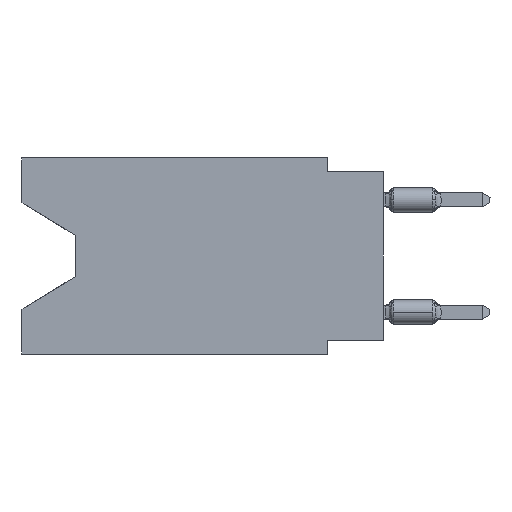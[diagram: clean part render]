
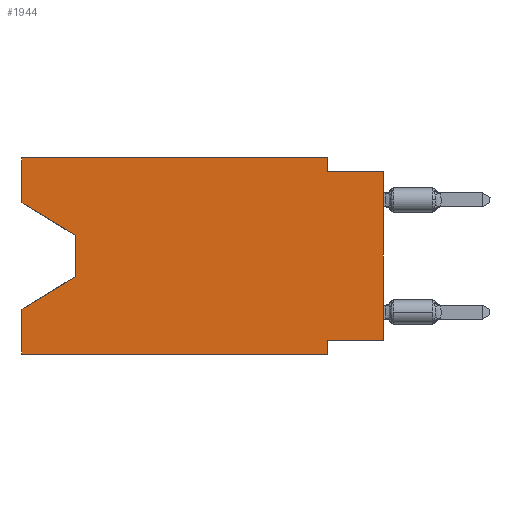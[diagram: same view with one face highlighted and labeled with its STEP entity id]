
A CAD part, left-side view. The second image highlights one B-rep face of the part: STEP entity #1944.
In plain terms, the highlighted planar face has unit normal (-1, 0, 0).
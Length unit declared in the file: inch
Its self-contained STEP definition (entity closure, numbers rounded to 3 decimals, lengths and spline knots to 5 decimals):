
#988 = VERTEX_POINT ( 'NONE', #22899 ) ;
#1447 = ORIENTED_EDGE ( 'NONE', *, *, #24468, .T. ) ;
#1481 = VECTOR ( 'NONE', #27851, 39.37008 ) ;
#1639 = CARTESIAN_POINT ( 'NONE',  ( 0., 0.645, 0. ) ) ;
#1944 = ADVANCED_FACE ( 'NONE', ( #41535 ), #12387, .F. ) ;
#2108 = DIRECTION ( 'NONE',  ( 0., 0., -1. ) ) ;
#2214 = CARTESIAN_POINT ( 'NONE',  ( 0., 0.1, -0.35 ) ) ;
#2319 = DIRECTION ( 'NONE',  ( 0., 0., 1. ) ) ;
#2640 = LINE ( 'NONE', #37544, #3293 ) ;
#3031 = CARTESIAN_POINT ( 'NONE',  ( 0., 0.645, -0.35 ) ) ;
#3290 = CARTESIAN_POINT ( 'NONE',  ( 0., 0.55, -0.212 ) ) ;
#3293 = VECTOR ( 'NONE', #4964, 39.37008 ) ;
#4300 = CARTESIAN_POINT ( 'NONE',  ( 0., 0.645, 0. ) ) ;
#4320 = ORIENTED_EDGE ( 'NONE', *, *, #34400, .T. ) ;
#4796 = VERTEX_POINT ( 'NONE', #3031 ) ;
#4964 = DIRECTION ( 'NONE',  ( 0., 0.855, -0.519 ) ) ;
#5058 = VECTOR ( 'NONE', #33320, 39.37008 ) ;
#5719 = VERTEX_POINT ( 'NONE', #34934 ) ;
#6164 = VERTEX_POINT ( 'NONE', #26337 ) ;
#6213 = ORIENTED_EDGE ( 'NONE', *, *, #31908, .T. ) ;
#6932 = VERTEX_POINT ( 'NONE', #9415 ) ;
#6958 = LINE ( 'NONE', #16128, #10249 ) ;
#6999 = EDGE_CURVE ( 'NONE', #37148, #988, #28565, .T. ) ;
#7096 = CARTESIAN_POINT ( 'NONE',  ( 0., 0., -0.325 ) ) ;
#7364 = EDGE_CURVE ( 'NONE', #4796, #14416, #20293, .T. ) ;
#7370 = EDGE_CURVE ( 'NONE', #6932, #6164, #36260, .T. ) ;
#7828 = ORIENTED_EDGE ( 'NONE', *, *, #25785, .F. ) ;
#8280 = LINE ( 'NONE', #27437, #1481 ) ;
#8325 = VECTOR ( 'NONE', #28193, 39.37008 ) ;
#8669 = LINE ( 'NONE', #1639, #30222 ) ;
#8988 = DIRECTION ( 'NONE',  ( 0., 0., -1. ) ) ;
#9415 = CARTESIAN_POINT ( 'NONE',  ( 0., 0., -0.325 ) ) ;
#9431 = AXIS2_PLACEMENT_3D ( 'NONE', #19007, #38139, #8988 ) ;
#9512 = CARTESIAN_POINT ( 'NONE',  ( 0., 0.55, -0.138 ) ) ;
#9664 = CARTESIAN_POINT ( 'NONE',  ( 0., 0.645, -0.26975 ) ) ;
#10249 = VECTOR ( 'NONE', #15926, 39.37008 ) ;
#11358 = CARTESIAN_POINT ( 'NONE',  ( 0., 0.1, 0. ) ) ;
#11545 = VERTEX_POINT ( 'NONE', #2214 ) ;
#12387 = PLANE ( 'NONE',  #9431 ) ;
#12395 = CARTESIAN_POINT ( 'NONE',  ( 0., 0.1, 0. ) ) ;
#12514 = ORIENTED_EDGE ( 'NONE', *, *, #12739, .F. ) ;
#12739 = EDGE_CURVE ( 'NONE', #6164, #11545, #18522, .T. ) ;
#13513 = ORIENTED_EDGE ( 'NONE', *, *, #7370, .F. ) ;
#14274 = VECTOR ( 'NONE', #25370, 39.37008 ) ;
#14416 = VERTEX_POINT ( 'NONE', #9664 ) ;
#15651 = EDGE_CURVE ( 'NONE', #35706, #37148, #8669, .T. ) ;
#15757 = VERTEX_POINT ( 'NONE', #9512 ) ;
#15847 = CARTESIAN_POINT ( 'NONE',  ( 0., 0.645, 0. ) ) ;
#15902 = EDGE_CURVE ( 'NONE', #988, #16058, #26734, .T. ) ;
#15926 = DIRECTION ( 'NONE',  ( 0., -1., 0. ) ) ;
#16058 = VERTEX_POINT ( 'NONE', #24145 ) ;
#16128 = CARTESIAN_POINT ( 'NONE',  ( 0., 0.645, -0.35 ) ) ;
#18515 = LINE ( 'NONE', #31475, #24544 ) ;
#18522 = LINE ( 'NONE', #21696, #28790 ) ;
#19007 = CARTESIAN_POINT ( 'NONE',  ( 0., 0.645, 0. ) ) ;
#19746 = VECTOR ( 'NONE', #30280, 39.37008 ) ;
#20093 = DIRECTION ( 'NONE',  ( 0., 1., 0. ) ) ;
#20208 = ORIENTED_EDGE ( 'NONE', *, *, #6999, .F. ) ;
#20293 = LINE ( 'NONE', #4300, #19746 ) ;
#20348 = CARTESIAN_POINT ( 'NONE',  ( 0., 0., -0.025 ) ) ;
#21696 = CARTESIAN_POINT ( 'NONE',  ( 0., 0.1, -0.35 ) ) ;
#22899 = CARTESIAN_POINT ( 'NONE',  ( 0., 0.1, -0.025 ) ) ;
#24094 = ORIENTED_EDGE ( 'NONE', *, *, #7364, .F. ) ;
#24145 = CARTESIAN_POINT ( 'NONE',  ( 0., 0., -0.025 ) ) ;
#24468 = EDGE_CURVE ( 'NONE', #5719, #15757, #27013, .T. ) ;
#24544 = VECTOR ( 'NONE', #2319, 39.37008 ) ;
#25370 = DIRECTION ( 'NONE',  ( 0., 0., -1. ) ) ;
#25597 = ORIENTED_EDGE ( 'NONE', *, *, #15902, .F. ) ;
#25785 = EDGE_CURVE ( 'NONE', #5719, #35706, #30972, .T. ) ;
#25956 = ORIENTED_EDGE ( 'NONE', *, *, #15651, .F. ) ;
#26337 = CARTESIAN_POINT ( 'NONE',  ( 0., 0.1, -0.325 ) ) ;
#26734 = LINE ( 'NONE', #20348, #5058 ) ;
#27013 = LINE ( 'NONE', #39998, #31681 ) ;
#27425 = DIRECTION ( 'NONE',  ( 0., -0.855, -0.519 ) ) ;
#27437 = CARTESIAN_POINT ( 'NONE',  ( 0., 0.55, -0.138 ) ) ;
#27850 = VECTOR ( 'NONE', #20093, 39.37008 ) ;
#27851 = DIRECTION ( 'NONE',  ( 0., 0., -1. ) ) ;
#28101 = EDGE_CURVE ( 'NONE', #4796, #11545, #6958, .T. ) ;
#28193 = DIRECTION ( 'NONE',  ( 0., 0., 1. ) ) ;
#28524 = VERTEX_POINT ( 'NONE', #3290 ) ;
#28565 = LINE ( 'NONE', #12395, #14274 ) ;
#28790 = VECTOR ( 'NONE', #2108, 39.37008 ) ;
#30222 = VECTOR ( 'NONE', #41219, 39.37008 ) ;
#30280 = DIRECTION ( 'NONE',  ( 0., 0., 1. ) ) ;
#30706 = EDGE_LOOP ( 'NONE', ( #1447, #6213, #4320, #24094, #39763, #12514, #13513, #37432, #25597, #20208, #25956, #7828 ) ) ;
#30972 = LINE ( 'NONE', #40769, #8325 ) ;
#31475 = CARTESIAN_POINT ( 'NONE',  ( 0., 0., 0. ) ) ;
#31681 = VECTOR ( 'NONE', #27425, 39.37008 ) ;
#31908 = EDGE_CURVE ( 'NONE', #15757, #28524, #8280, .T. ) ;
#33320 = DIRECTION ( 'NONE',  ( 0., -1., 0. ) ) ;
#34400 = EDGE_CURVE ( 'NONE', #28524, #14416, #2640, .T. ) ;
#34934 = CARTESIAN_POINT ( 'NONE',  ( 0., 0.645, -0.08025 ) ) ;
#35706 = VERTEX_POINT ( 'NONE', #15847 ) ;
#36260 = LINE ( 'NONE', #7096, #27850 ) ;
#37148 = VERTEX_POINT ( 'NONE', #11358 ) ;
#37432 = ORIENTED_EDGE ( 'NONE', *, *, #38162, .T. ) ;
#37544 = CARTESIAN_POINT ( 'NONE',  ( 0., 0.55, -0.212 ) ) ;
#38139 = DIRECTION ( 'NONE',  ( 1., 0., 0. ) ) ;
#38162 = EDGE_CURVE ( 'NONE', #6932, #16058, #18515, .T. ) ;
#39763 = ORIENTED_EDGE ( 'NONE', *, *, #28101, .T. ) ;
#39998 = CARTESIAN_POINT ( 'NONE',  ( 0., 0.645, -0.08025 ) ) ;
#40769 = CARTESIAN_POINT ( 'NONE',  ( 0., 0.645, 0. ) ) ;
#41219 = DIRECTION ( 'NONE',  ( 0., -1., 0. ) ) ;
#41535 = FACE_OUTER_BOUND ( 'NONE', #30706, .T. ) ;
